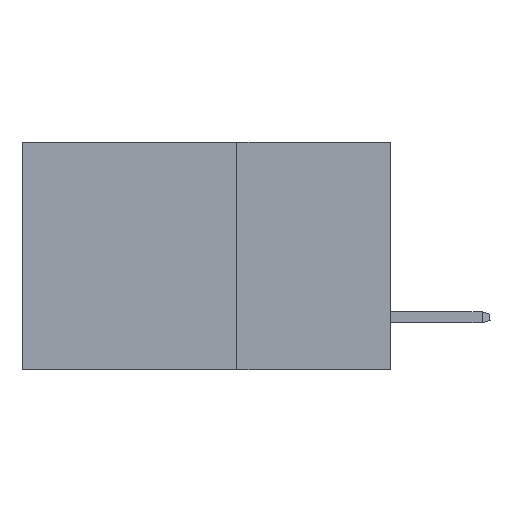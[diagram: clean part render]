
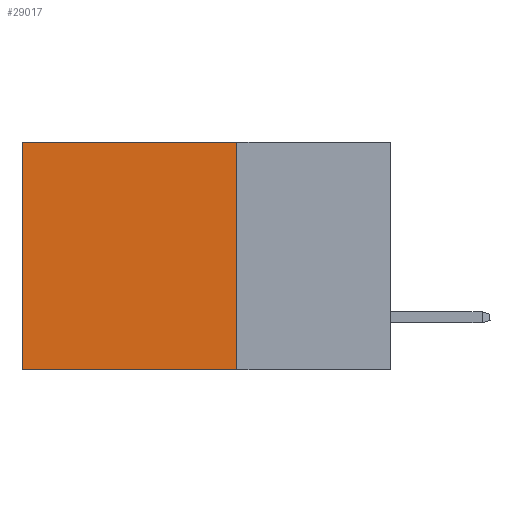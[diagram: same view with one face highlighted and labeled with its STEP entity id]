
A CAD part, left-side view. The second image highlights one B-rep face of the part: STEP entity #29017.
In plain terms, the highlighted planar face has unit normal (-1, 0, 0).
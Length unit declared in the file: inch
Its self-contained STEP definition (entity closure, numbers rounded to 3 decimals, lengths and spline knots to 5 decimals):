
#932 = AXIS2_PLACEMENT_3D ( 'NONE', #17412, #17637, #17891 ) ;
#4066 = CARTESIAN_POINT ( 'NONE',  ( 0.2875, 0.6, -0.37 ) ) ;
#4255 = ORIENTED_EDGE ( 'NONE', *, *, #20945, .T. ) ;
#4751 = VECTOR ( 'NONE', #15070, 39.37008 ) ;
#6414 = CARTESIAN_POINT ( 'NONE',  ( 0.2875, 0.6, 0. ) ) ;
#7169 = ORIENTED_EDGE ( 'NONE', *, *, #22152, .T. ) ;
#8370 = CARTESIAN_POINT ( 'NONE',  ( 0.2875, 0.25, 0. ) ) ;
#8518 = VECTOR ( 'NONE', #29481, 39.37008 ) ;
#8850 = VECTOR ( 'NONE', #17079, 39.37008 ) ;
#11981 = EDGE_LOOP ( 'NONE', ( #7169, #37145, #24007, #4255 ) ) ;
#14165 = LINE ( 'NONE', #6414, #4751 ) ;
#14543 = PLANE ( 'NONE',  #932 ) ;
#15070 = DIRECTION ( 'NONE',  ( 0., 0., -1. ) ) ;
#15096 = VERTEX_POINT ( 'NONE', #4066 ) ;
#16121 = LINE ( 'NONE', #29753, #8518 ) ;
#16180 = EDGE_CURVE ( 'NONE', #31239, #15096, #16121, .T. ) ;
#16940 = LINE ( 'NONE', #8370, #8850 ) ;
#17079 = DIRECTION ( 'NONE',  ( 0., 1., 0. ) ) ;
#17287 = VECTOR ( 'NONE', #28782, 39.37008 ) ;
#17412 = CARTESIAN_POINT ( 'NONE',  ( 0.2875, 0.25, 0. ) ) ;
#17555 = EDGE_CURVE ( 'NONE', #29676, #31239, #32999, .T. ) ;
#17637 = DIRECTION ( 'NONE',  ( 1., 0., 0. ) ) ;
#17891 = DIRECTION ( 'NONE',  ( 0., 0., -1. ) ) ;
#18145 = VERTEX_POINT ( 'NONE', #20560 ) ;
#20560 = CARTESIAN_POINT ( 'NONE',  ( 0.2875, 0.6, 0. ) ) ;
#20945 = EDGE_CURVE ( 'NONE', #29676, #18145, #16940, .T. ) ;
#22152 = EDGE_CURVE ( 'NONE', #18145, #15096, #14165, .T. ) ;
#22961 = CARTESIAN_POINT ( 'NONE',  ( 0.2875, 0.25, 0. ) ) ;
#24007 = ORIENTED_EDGE ( 'NONE', *, *, #17555, .F. ) ;
#28782 = DIRECTION ( 'NONE',  ( 0., 0., -1. ) ) ;
#29017 = ADVANCED_FACE ( 'NONE', ( #29043 ), #14543, .F. ) ;
#29043 = FACE_OUTER_BOUND ( 'NONE', #11981, .T. ) ;
#29251 = CARTESIAN_POINT ( 'NONE',  ( 0.2875, 0.25, -0.37 ) ) ;
#29481 = DIRECTION ( 'NONE',  ( 0., 1., 0. ) ) ;
#29676 = VERTEX_POINT ( 'NONE', #31604 ) ;
#29753 = CARTESIAN_POINT ( 'NONE',  ( 0.2875, 0.25, -0.37 ) ) ;
#31239 = VERTEX_POINT ( 'NONE', #29251 ) ;
#31604 = CARTESIAN_POINT ( 'NONE',  ( 0.2875, 0.25, 0. ) ) ;
#32999 = LINE ( 'NONE', #22961, #17287 ) ;
#37145 = ORIENTED_EDGE ( 'NONE', *, *, #16180, .F. ) ;
